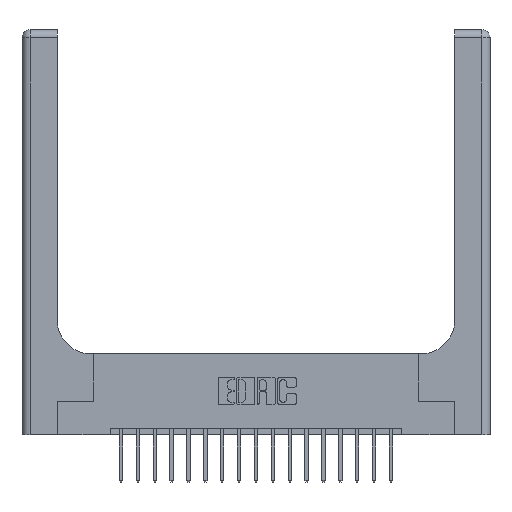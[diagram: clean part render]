
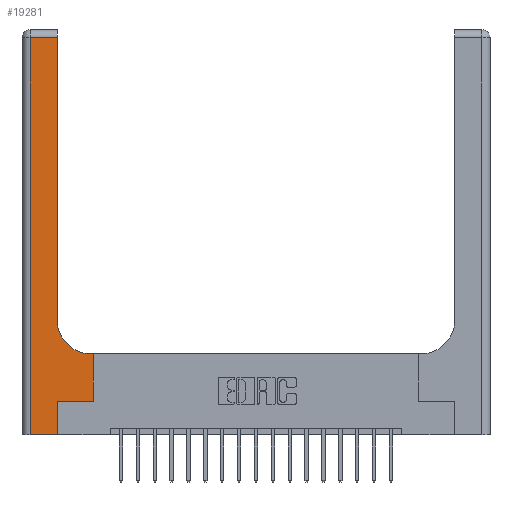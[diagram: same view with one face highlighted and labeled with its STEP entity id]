
A CAD part, top view. The second image highlights one B-rep face of the part: STEP entity #19281.
In plain terms, the highlighted planar face has unit normal (0, 0, 1).
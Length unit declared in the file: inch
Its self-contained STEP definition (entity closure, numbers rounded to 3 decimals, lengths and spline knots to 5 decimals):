
#21 = VERTEX_POINT ( 'NONE', #2901 ) ;
#48 = DIRECTION ( 'NONE',  ( 0., -1., 0. ) ) ;
#130 = CARTESIAN_POINT ( 'NONE',  ( 0.528, 0.25, 0.37 ) ) ;
#175 = AXIS2_PLACEMENT_3D ( 'NONE', #5954, #16551, #12006 ) ;
#291 = ORIENTED_EDGE ( 'NONE', *, *, #11784, .T. ) ;
#1351 = CARTESIAN_POINT ( 'NONE',  ( 0., 2.94, 0.37 ) ) ;
#1573 = EDGE_LOOP ( 'NONE', ( #12011, #4611, #17374, #291, #14087, #4547, #3443, #6168, #14860 ) ) ;
#1627 = LINE ( 'NONE', #10790, #2832 ) ;
#1742 = CARTESIAN_POINT ( 'NONE',  ( 0.265, 0.25, 0.37 ) ) ;
#1771 = DIRECTION ( 'NONE',  ( -1., 0., 0. ) ) ;
#2223 = CARTESIAN_POINT ( 'NONE',  ( 0.26, 0.6, 0.37 ) ) ;
#2292 = VERTEX_POINT ( 'NONE', #15825 ) ;
#2329 = LINE ( 'NONE', #9038, #15607 ) ;
#2495 = VERTEX_POINT ( 'NONE', #13094 ) ;
#2643 = DIRECTION ( 'NONE',  ( -1., 0., 0. ) ) ;
#2832 = VECTOR ( 'NONE', #4973, 39.37008 ) ;
#2901 = CARTESIAN_POINT ( 'NONE',  ( 0.06, 2.94, 0.37 ) ) ;
#3099 = CARTESIAN_POINT ( 'NONE',  ( 0.265, 0.25, 0.37 ) ) ;
#3296 = VERTEX_POINT ( 'NONE', #19595 ) ;
#3443 = ORIENTED_EDGE ( 'NONE', *, *, #13743, .T. ) ;
#3489 = EDGE_CURVE ( 'NONE', #2495, #19368, #9684, .T. ) ;
#4048 = VECTOR ( 'NONE', #48, 39.37008 ) ;
#4125 = VERTEX_POINT ( 'NONE', #3099 ) ;
#4298 = VECTOR ( 'NONE', #18398, 39.37008 ) ;
#4547 = ORIENTED_EDGE ( 'NONE', *, *, #13941, .T. ) ;
#4611 = ORIENTED_EDGE ( 'NONE', *, *, #11597, .T. ) ;
#4918 = EDGE_CURVE ( 'NONE', #19368, #2292, #11996, .T. ) ;
#4973 = DIRECTION ( 'NONE',  ( 1., 0., 0. ) ) ;
#5009 = FACE_OUTER_BOUND ( 'NONE', #1573, .T. ) ;
#5388 = VECTOR ( 'NONE', #6702, 39.37008 ) ;
#5954 = CARTESIAN_POINT ( 'NONE',  ( 0.51, 0.85, 0.37 ) ) ;
#6168 = ORIENTED_EDGE ( 'NONE', *, *, #3489, .T. ) ;
#6244 = DIRECTION ( 'NONE',  ( 0., 1., 0. ) ) ;
#6375 = DIRECTION ( 'NONE',  ( 1., 0., 0. ) ) ;
#6702 = DIRECTION ( 'NONE',  ( -1., 0., 0. ) ) ;
#6920 = LINE ( 'NONE', #13817, #4048 ) ;
#7683 = VERTEX_POINT ( 'NONE', #130 ) ;
#7790 = VECTOR ( 'NONE', #6375, 39.37008 ) ;
#7851 = CARTESIAN_POINT ( 'NONE',  ( 0.26, 3., 0.37 ) ) ;
#9038 = CARTESIAN_POINT ( 'NONE',  ( 0.528, 0.25, 0.37 ) ) ;
#9191 = CARTESIAN_POINT ( 'NONE',  ( 0., 3., 0.37 ) ) ;
#9655 = VERTEX_POINT ( 'NONE', #15227 ) ;
#9684 = LINE ( 'NONE', #2223, #5388 ) ;
#10386 = VECTOR ( 'NONE', #12003, 39.37008 ) ;
#10626 = PLANE ( 'NONE',  #15856 ) ;
#10790 = CARTESIAN_POINT ( 'NONE',  ( 0., 0., 0.37 ) ) ;
#11597 = EDGE_CURVE ( 'NONE', #9655, #21, #13257, .T. ) ;
#11784 = EDGE_CURVE ( 'NONE', #13932, #3296, #1627, .T. ) ;
#11996 = CIRCLE ( 'NONE', #175, 0.25 ) ;
#12003 = DIRECTION ( 'NONE',  ( 0., 1., 0. ) ) ;
#12006 = DIRECTION ( 'NONE',  ( 1., 0., 0. ) ) ;
#12011 = ORIENTED_EDGE ( 'NONE', *, *, #18299, .T. ) ;
#12264 = LINE ( 'NONE', #7851, #4298 ) ;
#12387 = DIRECTION ( 'NONE',  ( 0., 0., -1. ) ) ;
#12924 = LINE ( 'NONE', #1742, #7790 ) ;
#13094 = CARTESIAN_POINT ( 'NONE',  ( 0.528, 0.6, 0.37 ) ) ;
#13257 = LINE ( 'NONE', #1351, #16874 ) ;
#13691 = CARTESIAN_POINT ( 'NONE',  ( 0.51, 0.6, 0.37 ) ) ;
#13743 = EDGE_CURVE ( 'NONE', #7683, #2495, #2329, .T. ) ;
#13817 = CARTESIAN_POINT ( 'NONE',  ( 0.06, 3., 0.37 ) ) ;
#13932 = VERTEX_POINT ( 'NONE', #15676 ) ;
#13941 = EDGE_CURVE ( 'NONE', #4125, #7683, #12924, .T. ) ;
#14087 = ORIENTED_EDGE ( 'NONE', *, *, #18307, .T. ) ;
#14860 = ORIENTED_EDGE ( 'NONE', *, *, #4918, .T. ) ;
#15119 = CARTESIAN_POINT ( 'NONE',  ( 0.265, 0., 0.37 ) ) ;
#15227 = CARTESIAN_POINT ( 'NONE',  ( 0.26, 2.94, 0.37 ) ) ;
#15607 = VECTOR ( 'NONE', #6244, 39.37008 ) ;
#15676 = CARTESIAN_POINT ( 'NONE',  ( 0.06, 0., 0.37 ) ) ;
#15825 = CARTESIAN_POINT ( 'NONE',  ( 0.26, 0.85, 0.37 ) ) ;
#15856 = AXIS2_PLACEMENT_3D ( 'NONE', #9191, #12387, #1771 ) ;
#16551 = DIRECTION ( 'NONE',  ( 0., 0., -1. ) ) ;
#16874 = VECTOR ( 'NONE', #2643, 39.37008 ) ;
#17374 = ORIENTED_EDGE ( 'NONE', *, *, #19257, .T. ) ;
#17569 = LINE ( 'NONE', #15119, #10386 ) ;
#18299 = EDGE_CURVE ( 'NONE', #2292, #9655, #12264, .T. ) ;
#18307 = EDGE_CURVE ( 'NONE', #3296, #4125, #17569, .T. ) ;
#18398 = DIRECTION ( 'NONE',  ( 0., 1., 0. ) ) ;
#19257 = EDGE_CURVE ( 'NONE', #21, #13932, #6920, .T. ) ;
#19281 = ADVANCED_FACE ( 'NONE', ( #5009 ), #10626, .F. ) ;
#19368 = VERTEX_POINT ( 'NONE', #13691 ) ;
#19595 = CARTESIAN_POINT ( 'NONE',  ( 0.265, 0., 0.37 ) ) ;
